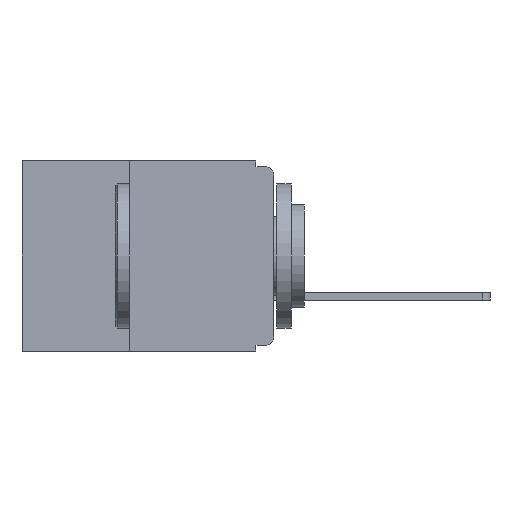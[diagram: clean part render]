
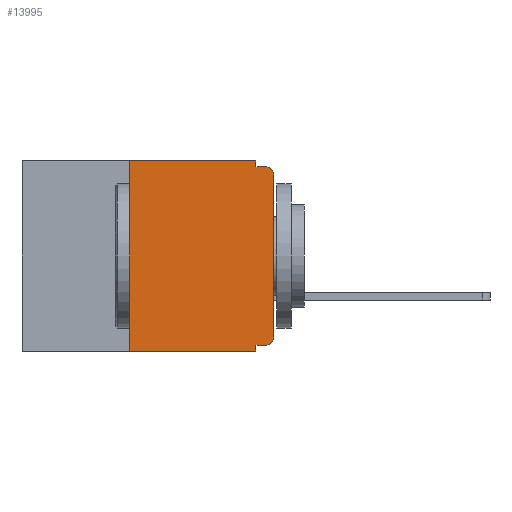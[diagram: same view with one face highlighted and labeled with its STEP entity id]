
A CAD part, left-side view. The second image highlights one B-rep face of the part: STEP entity #13995.
In plain terms, the highlighted planar face has unit normal (-1, 0, 0).
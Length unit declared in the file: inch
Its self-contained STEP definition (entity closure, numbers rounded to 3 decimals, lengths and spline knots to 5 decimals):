
#700 = LINE ( 'NONE', #4170, #24240 ) ;
#745 = VECTOR ( 'NONE', #14140, 39.37008 ) ;
#813 = ORIENTED_EDGE ( 'NONE', *, *, #20309, .F. ) ;
#854 = CARTESIAN_POINT ( 'NONE',  ( 0., 0.25, -0.33 ) ) ;
#1791 = LINE ( 'NONE', #14623, #12231 ) ;
#1874 = EDGE_CURVE ( 'NONE', #7683, #14372, #27178, .T. ) ;
#2513 = CARTESIAN_POINT ( 'NONE',  ( 0., 0., 0. ) ) ;
#3168 = VECTOR ( 'NONE', #11452, 39.37008 ) ;
#3444 = CARTESIAN_POINT ( 'NONE',  ( 0., 0.437, -0.33 ) ) ;
#3612 = DIRECTION ( 'NONE',  ( 0., 1., 0. ) ) ;
#3786 = PLANE ( 'NONE',  #9204 ) ;
#3918 = VECTOR ( 'NONE', #22695, 39.37008 ) ;
#4170 = CARTESIAN_POINT ( 'NONE',  ( 0., 0.437, 0. ) ) ;
#4493 = CARTESIAN_POINT ( 'NONE',  ( 0., 0.031, -0.33 ) ) ;
#4533 = DIRECTION ( 'NONE',  ( -1., 0., 0. ) ) ;
#4903 = VERTEX_POINT ( 'NONE', #16888 ) ;
#5928 = LINE ( 'NONE', #2513, #3168 ) ;
#6413 = EDGE_CURVE ( 'NONE', #23146, #21572, #1791, .T. ) ;
#6699 = EDGE_CURVE ( 'NONE', #23146, #10687, #12371, .T. ) ;
#7386 = CARTESIAN_POINT ( 'NONE',  ( 0., 0.015, -0.025 ) ) ;
#7683 = VERTEX_POINT ( 'NONE', #12541 ) ;
#8468 = CARTESIAN_POINT ( 'NONE',  ( 0., 0.031, -0.33 ) ) ;
#8886 = EDGE_LOOP ( 'NONE', ( #28551, #15895, #21474, #12882, #17125, #9188, #25331, #813, #11951, #12324 ) ) ;
#9188 = ORIENTED_EDGE ( 'NONE', *, *, #20993, .F. ) ;
#9204 = AXIS2_PLACEMENT_3D ( 'NONE', #23686, #12703, #28023 ) ;
#9613 = EDGE_CURVE ( 'NONE', #14372, #27026, #20126, .T. ) ;
#9634 = DIRECTION ( 'NONE',  ( 0., 0., -1. ) ) ;
#9669 = VECTOR ( 'NONE', #17326, 39.37008 ) ;
#9828 = LINE ( 'NONE', #3444, #3918 ) ;
#10687 = VERTEX_POINT ( 'NONE', #22359 ) ;
#11166 = CARTESIAN_POINT ( 'NONE',  ( 0., 0.015, -0.32 ) ) ;
#11368 = CARTESIAN_POINT ( 'NONE',  ( 0., 0.015, -0.01 ) ) ;
#11452 = DIRECTION ( 'NONE',  ( 0., 0., 1. ) ) ;
#11725 = CARTESIAN_POINT ( 'NONE',  ( 0., 0.031, -0.32 ) ) ;
#11782 = VERTEX_POINT ( 'NONE', #8468 ) ;
#11941 = CARTESIAN_POINT ( 'NONE',  ( 0., 0., -0.01 ) ) ;
#11951 = ORIENTED_EDGE ( 'NONE', *, *, #6413, .F. ) ;
#12231 = VECTOR ( 'NONE', #3612, 39.37008 ) ;
#12324 = ORIENTED_EDGE ( 'NONE', *, *, #6699, .T. ) ;
#12371 = CIRCLE ( 'NONE', #27444, 0.015 ) ;
#12541 = CARTESIAN_POINT ( 'NONE',  ( 0., 0.031, 0. ) ) ;
#12703 = DIRECTION ( 'NONE',  ( 1., 0., 0. ) ) ;
#12882 = ORIENTED_EDGE ( 'NONE', *, *, #1874, .F. ) ;
#12957 = LINE ( 'NONE', #4493, #23982 ) ;
#13066 = CARTESIAN_POINT ( 'NONE',  ( 0., 0.25, -0.33 ) ) ;
#13319 = DIRECTION ( 'NONE',  ( 0., 0., -1. ) ) ;
#13995 = ADVANCED_FACE ( 'NONE', ( #24981 ), #3786, .F. ) ;
#14140 = DIRECTION ( 'NONE',  ( 0., 0., 1. ) ) ;
#14228 = VECTOR ( 'NONE', #23008, 39.37008 ) ;
#14372 = VERTEX_POINT ( 'NONE', #16247 ) ;
#14623 = CARTESIAN_POINT ( 'NONE',  ( 0., 0., -0.32 ) ) ;
#14937 = VERTEX_POINT ( 'NONE', #13066 ) ;
#14984 = EDGE_CURVE ( 'NONE', #10687, #4903, #5928, .T. ) ;
#15895 = ORIENTED_EDGE ( 'NONE', *, *, #28391, .T. ) ;
#15922 = VERTEX_POINT ( 'NONE', #27766 ) ;
#16247 = CARTESIAN_POINT ( 'NONE',  ( 0., 0.031, -0.01 ) ) ;
#16888 = CARTESIAN_POINT ( 'NONE',  ( 0., 0., -0.025 ) ) ;
#17125 = ORIENTED_EDGE ( 'NONE', *, *, #26880, .F. ) ;
#17326 = DIRECTION ( 'NONE',  ( 0., 0., -1. ) ) ;
#17809 = CARTESIAN_POINT ( 'NONE',  ( 0., 0.015, -0.305 ) ) ;
#20037 = DIRECTION ( 'NONE',  ( 0., 0., -1. ) ) ;
#20126 = LINE ( 'NONE', #11941, #14228 ) ;
#20309 = EDGE_CURVE ( 'NONE', #21572, #11782, #12957, .T. ) ;
#20653 = EDGE_CURVE ( 'NONE', #14937, #11782, #9828, .T. ) ;
#20993 = EDGE_CURVE ( 'NONE', #14937, #15922, #21232, .T. ) ;
#21232 = LINE ( 'NONE', #854, #745 ) ;
#21474 = ORIENTED_EDGE ( 'NONE', *, *, #9613, .F. ) ;
#21572 = VERTEX_POINT ( 'NONE', #11725 ) ;
#22359 = CARTESIAN_POINT ( 'NONE',  ( 0., 0., -0.305 ) ) ;
#22695 = DIRECTION ( 'NONE',  ( 0., -1., 0. ) ) ;
#22848 = DIRECTION ( 'NONE',  ( -1., 0., 0. ) ) ;
#23008 = DIRECTION ( 'NONE',  ( 0., -1., 0. ) ) ;
#23146 = VERTEX_POINT ( 'NONE', #11166 ) ;
#23686 = CARTESIAN_POINT ( 'NONE',  ( 0., 0.437, 0. ) ) ;
#23979 = DIRECTION ( 'NONE',  ( 0., -1., 0. ) ) ;
#23982 = VECTOR ( 'NONE', #13319, 39.37008 ) ;
#24240 = VECTOR ( 'NONE', #23979, 39.37008 ) ;
#24845 = CARTESIAN_POINT ( 'NONE',  ( 0., 0.031, 0. ) ) ;
#24981 = FACE_OUTER_BOUND ( 'NONE', #8886, .T. ) ;
#25331 = ORIENTED_EDGE ( 'NONE', *, *, #20653, .T. ) ;
#26023 = AXIS2_PLACEMENT_3D ( 'NONE', #7386, #22848, #9634 ) ;
#26880 = EDGE_CURVE ( 'NONE', #15922, #7683, #700, .T. ) ;
#27026 = VERTEX_POINT ( 'NONE', #11368 ) ;
#27178 = LINE ( 'NONE', #24845, #9669 ) ;
#27444 = AXIS2_PLACEMENT_3D ( 'NONE', #17809, #4533, #20037 ) ;
#27766 = CARTESIAN_POINT ( 'NONE',  ( 0., 0.25, 0. ) ) ;
#28023 = DIRECTION ( 'NONE',  ( 0., 0., -1. ) ) ;
#28193 = CIRCLE ( 'NONE', #26023, 0.015 ) ;
#28391 = EDGE_CURVE ( 'NONE', #4903, #27026, #28193, .T. ) ;
#28551 = ORIENTED_EDGE ( 'NONE', *, *, #14984, .T. ) ;
